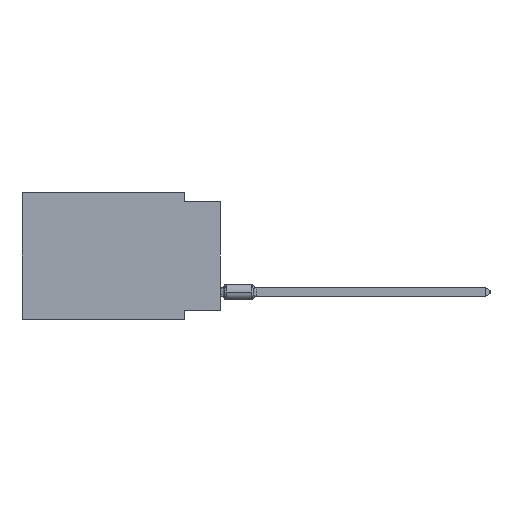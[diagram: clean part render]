
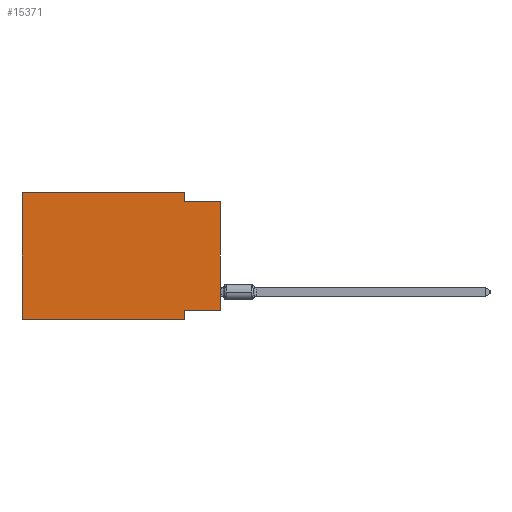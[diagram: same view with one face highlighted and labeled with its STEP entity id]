
A CAD part, left-side view. The second image highlights one B-rep face of the part: STEP entity #15371.
In plain terms, the highlighted planar face has unit normal (-1, 0, 0).
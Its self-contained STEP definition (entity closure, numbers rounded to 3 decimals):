
#678 = CARTESIAN_POINT ( 'NONE',  ( 0., 0., -8.255 ) ) ;
#983 = VERTEX_POINT ( 'NONE', #3209 ) ;
#1422 = VERTEX_POINT ( 'NONE', #12215 ) ;
#1473 = LINE ( 'NONE', #3988, #9513 ) ;
#1880 = DIRECTION ( 'NONE',  ( 1., 0., 0. ) ) ;
#2347 = VERTEX_POINT ( 'NONE', #8578 ) ;
#2358 = EDGE_LOOP ( 'NONE', ( #11278, #8322, #8575, #13347, #11679, #6266, #11748, #15079 ) ) ;
#2643 = EDGE_CURVE ( 'NONE', #9428, #10540, #2892, .T. ) ;
#2892 = LINE ( 'NONE', #11036, #13220 ) ;
#3209 = CARTESIAN_POINT ( 'NONE',  ( 0., 2.54, -8.255 ) ) ;
#3244 = DIRECTION ( 'NONE',  ( 0., -1., 0. ) ) ;
#3636 = CARTESIAN_POINT ( 'NONE',  ( 0., 13.97, -8.89 ) ) ;
#3748 = CARTESIAN_POINT ( 'NONE',  ( 0., 2.54, -8.89 ) ) ;
#3799 = EDGE_CURVE ( 'NONE', #7220, #10540, #5584, .T. ) ;
#3954 = EDGE_CURVE ( 'NONE', #983, #4825, #10075, .T. ) ;
#3988 = CARTESIAN_POINT ( 'NONE',  ( 0., 13.97, 0. ) ) ;
#4001 = EDGE_CURVE ( 'NONE', #2347, #1422, #1473, .T. ) ;
#4473 = PLANE ( 'NONE',  #12780 ) ;
#4536 = VECTOR ( 'NONE', #4826, 1000. ) ;
#4825 = VERTEX_POINT ( 'NONE', #16484 ) ;
#4826 = DIRECTION ( 'NONE',  ( 0., 1., 0. ) ) ;
#4897 = DIRECTION ( 'NONE',  ( 0., -1., 0. ) ) ;
#4909 = LINE ( 'NONE', #15082, #6208 ) ;
#5399 = CARTESIAN_POINT ( 'NONE',  ( 0., 2.54, -0.635 ) ) ;
#5584 = LINE ( 'NONE', #14528, #6606 ) ;
#5633 = VECTOR ( 'NONE', #16463, 1000. ) ;
#6207 = EDGE_CURVE ( 'NONE', #9428, #983, #7156, .T. ) ;
#6208 = VECTOR ( 'NONE', #4897, 1000. ) ;
#6266 = ORIENTED_EDGE ( 'NONE', *, *, #7331, .T. ) ;
#6606 = VECTOR ( 'NONE', #3244, 1000. ) ;
#6891 = DIRECTION ( 'NONE',  ( 0., 0., -1. ) ) ;
#7156 = LINE ( 'NONE', #9733, #4536 ) ;
#7220 = VERTEX_POINT ( 'NONE', #5399 ) ;
#7331 = EDGE_CURVE ( 'NONE', #2347, #4825, #10970, .T. ) ;
#7666 = VECTOR ( 'NONE', #8576, 1000. ) ;
#8322 = ORIENTED_EDGE ( 'NONE', *, *, #3799, .F. ) ;
#8575 = ORIENTED_EDGE ( 'NONE', *, *, #8653, .F. ) ;
#8576 = DIRECTION ( 'NONE',  ( 0., 0., -1. ) ) ;
#8578 = CARTESIAN_POINT ( 'NONE',  ( 0., 13.97, -8.89 ) ) ;
#8653 = EDGE_CURVE ( 'NONE', #12722, #7220, #14207, .T. ) ;
#8763 = CARTESIAN_POINT ( 'NONE',  ( 0., 2.54, 0. ) ) ;
#9299 = FACE_OUTER_BOUND ( 'NONE', #2358, .T. ) ;
#9428 = VERTEX_POINT ( 'NONE', #678 ) ;
#9458 = EDGE_CURVE ( 'NONE', #1422, #12722, #4909, .T. ) ;
#9513 = VECTOR ( 'NONE', #14259, 1000. ) ;
#9597 = VECTOR ( 'NONE', #14833, 1000. ) ;
#9733 = CARTESIAN_POINT ( 'NONE',  ( 0., 0., -8.255 ) ) ;
#10075 = LINE ( 'NONE', #3748, #7666 ) ;
#10540 = VERTEX_POINT ( 'NONE', #14136 ) ;
#10943 = CARTESIAN_POINT ( 'NONE',  ( 0., 2.54, 0. ) ) ;
#10970 = LINE ( 'NONE', #3636, #9597 ) ;
#11036 = CARTESIAN_POINT ( 'NONE',  ( 0., 0., 0. ) ) ;
#11278 = ORIENTED_EDGE ( 'NONE', *, *, #2643, .T. ) ;
#11679 = ORIENTED_EDGE ( 'NONE', *, *, #4001, .F. ) ;
#11748 = ORIENTED_EDGE ( 'NONE', *, *, #3954, .F. ) ;
#12215 = CARTESIAN_POINT ( 'NONE',  ( 0., 13.97, 0. ) ) ;
#12722 = VERTEX_POINT ( 'NONE', #10943 ) ;
#12780 = AXIS2_PLACEMENT_3D ( 'NONE', #13245, #1880, #6891 ) ;
#13220 = VECTOR ( 'NONE', #14653, 1000. ) ;
#13245 = CARTESIAN_POINT ( 'NONE',  ( 0., 13.97, 0. ) ) ;
#13347 = ORIENTED_EDGE ( 'NONE', *, *, #9458, .F. ) ;
#14136 = CARTESIAN_POINT ( 'NONE',  ( 0., 0., -0.635 ) ) ;
#14207 = LINE ( 'NONE', #8763, #5633 ) ;
#14259 = DIRECTION ( 'NONE',  ( 0., 0., 1. ) ) ;
#14528 = CARTESIAN_POINT ( 'NONE',  ( 0., 0., -0.635 ) ) ;
#14653 = DIRECTION ( 'NONE',  ( 0., 0., 1. ) ) ;
#14833 = DIRECTION ( 'NONE',  ( 0., -1., 0. ) ) ;
#15079 = ORIENTED_EDGE ( 'NONE', *, *, #6207, .F. ) ;
#15082 = CARTESIAN_POINT ( 'NONE',  ( 0., 13.97, 0. ) ) ;
#15371 = ADVANCED_FACE ( 'NONE', ( #9299 ), #4473, .F. ) ;
#16463 = DIRECTION ( 'NONE',  ( 0., 0., -1. ) ) ;
#16484 = CARTESIAN_POINT ( 'NONE',  ( 0., 2.54, -8.89 ) ) ;
